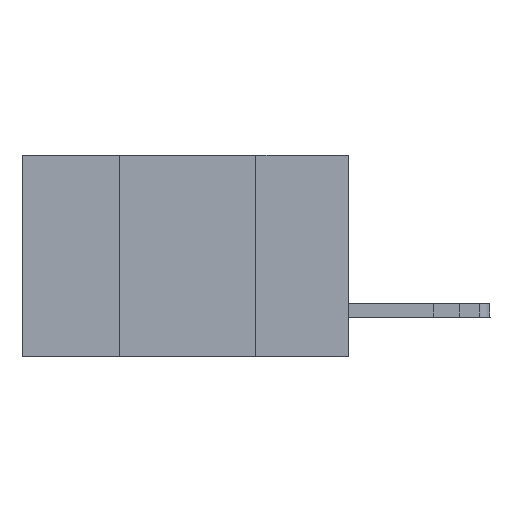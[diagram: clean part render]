
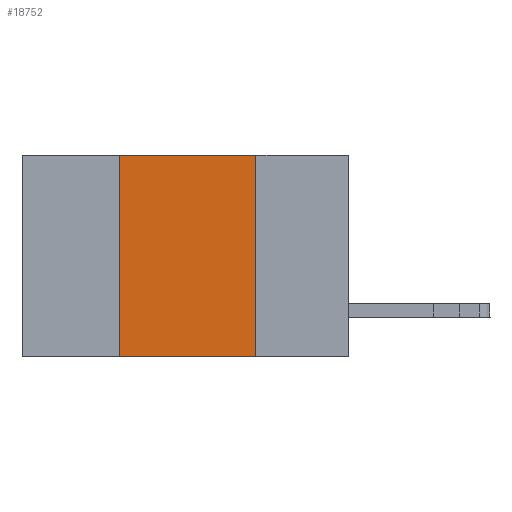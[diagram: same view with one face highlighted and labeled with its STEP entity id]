
A CAD part, left-side view. The second image highlights one B-rep face of the part: STEP entity #18752.
In plain terms, the highlighted planar face has unit normal (-1, 0, 0).
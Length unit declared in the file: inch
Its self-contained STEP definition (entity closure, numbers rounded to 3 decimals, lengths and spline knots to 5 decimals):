
#136 = EDGE_CURVE ( 'NONE', #10138, #22886, #16598, .T. ) ;
#245 = ORIENTED_EDGE ( 'NONE', *, *, #136, .F. ) ;
#768 = VECTOR ( 'NONE', #18024, 39.37008 ) ;
#1706 = CARTESIAN_POINT ( 'NONE',  ( 0., 0.42, 0. ) ) ;
#1906 = CARTESIAN_POINT ( 'NONE',  ( 0., 0.6, 0. ) ) ;
#2558 = LINE ( 'NONE', #7908, #8899 ) ;
#3430 = VERTEX_POINT ( 'NONE', #15829 ) ;
#3558 = ORIENTED_EDGE ( 'NONE', *, *, #16899, .F. ) ;
#6067 = CARTESIAN_POINT ( 'NONE',  ( 0., 0.6, 0. ) ) ;
#6833 = VECTOR ( 'NONE', #13411, 39.37008 ) ;
#7507 = DIRECTION ( 'NONE',  ( 0., 0., -1. ) ) ;
#7908 = CARTESIAN_POINT ( 'NONE',  ( 0., 0.6, -0.37 ) ) ;
#8858 = LINE ( 'NONE', #1706, #768 ) ;
#8899 = VECTOR ( 'NONE', #20445, 39.37008 ) ;
#9341 = AXIS2_PLACEMENT_3D ( 'NONE', #1906, #22687, #7507 ) ;
#10056 = EDGE_LOOP ( 'NONE', ( #245, #16197, #3558, #12590 ) ) ;
#10138 = VERTEX_POINT ( 'NONE', #11713 ) ;
#11705 = EDGE_CURVE ( 'NONE', #3430, #10138, #20545, .T. ) ;
#11713 = CARTESIAN_POINT ( 'NONE',  ( 0., 0.17, 0. ) ) ;
#12590 = ORIENTED_EDGE ( 'NONE', *, *, #16588, .T. ) ;
#13411 = DIRECTION ( 'NONE',  ( 0., -1., 0. ) ) ;
#14610 = FACE_OUTER_BOUND ( 'NONE', #10056, .T. ) ;
#15151 = CARTESIAN_POINT ( 'NONE',  ( 0., 0.17, -0.37 ) ) ;
#15829 = CARTESIAN_POINT ( 'NONE',  ( 0., 0.42, 0. ) ) ;
#16197 = ORIENTED_EDGE ( 'NONE', *, *, #11705, .F. ) ;
#16588 = EDGE_CURVE ( 'NONE', #21865, #22886, #2558, .T. ) ;
#16598 = LINE ( 'NONE', #20216, #18124 ) ;
#16899 = EDGE_CURVE ( 'NONE', #21865, #3430, #8858, .T. ) ;
#18024 = DIRECTION ( 'NONE',  ( 0., 0., 1. ) ) ;
#18122 = CARTESIAN_POINT ( 'NONE',  ( 0., 0.42, -0.37 ) ) ;
#18124 = VECTOR ( 'NONE', #18877, 39.37008 ) ;
#18752 = ADVANCED_FACE ( 'NONE', ( #14610 ), #21971, .F. ) ;
#18877 = DIRECTION ( 'NONE',  ( 0., 0., -1. ) ) ;
#20216 = CARTESIAN_POINT ( 'NONE',  ( 0., 0.17, 0. ) ) ;
#20445 = DIRECTION ( 'NONE',  ( 0., -1., 0. ) ) ;
#20545 = LINE ( 'NONE', #6067, #6833 ) ;
#21865 = VERTEX_POINT ( 'NONE', #18122 ) ;
#21971 = PLANE ( 'NONE',  #9341 ) ;
#22687 = DIRECTION ( 'NONE',  ( 1., 0., 0. ) ) ;
#22886 = VERTEX_POINT ( 'NONE', #15151 ) ;
